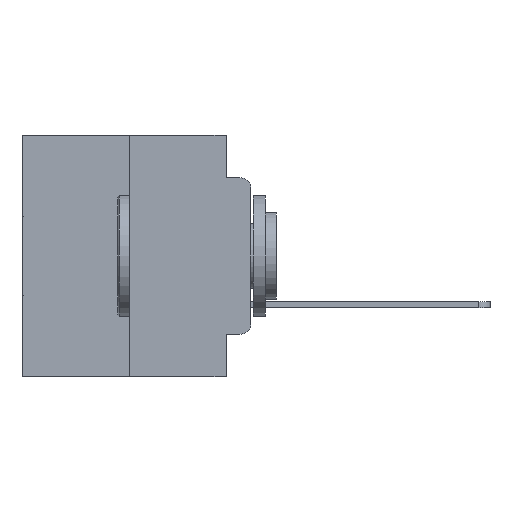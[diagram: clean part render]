
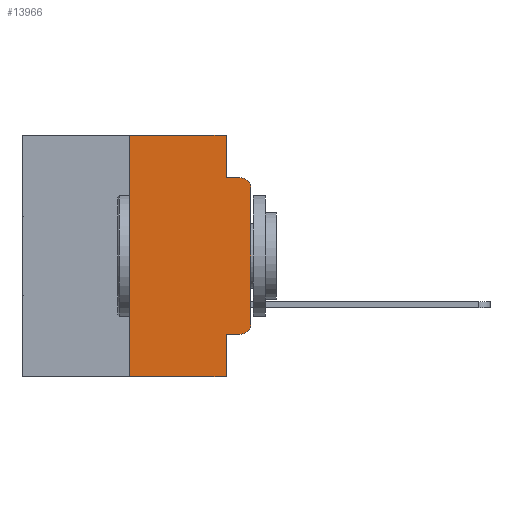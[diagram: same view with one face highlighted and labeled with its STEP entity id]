
A CAD part, left-side view. The second image highlights one B-rep face of the part: STEP entity #13966.
In plain terms, the highlighted planar face has unit normal (-1, 0, 0).
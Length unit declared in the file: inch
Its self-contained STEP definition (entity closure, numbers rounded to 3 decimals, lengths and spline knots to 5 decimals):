
#57 = VECTOR ( 'NONE', #1655, 39.37008 ) ;
#289 = CARTESIAN_POINT ( 'NONE',  ( 0., 0.051, 0. ) ) ;
#354 = DIRECTION ( 'NONE',  ( 1., 0., 0. ) ) ;
#413 = VERTEX_POINT ( 'NONE', #11187 ) ;
#441 = ORIENTED_EDGE ( 'NONE', *, *, #23303, .F. ) ;
#839 = EDGE_CURVE ( 'NONE', #23114, #413, #25658, .T. ) ;
#843 = VERTEX_POINT ( 'NONE', #8061 ) ;
#1576 = CARTESIAN_POINT ( 'NONE',  ( 0., 0., -0.3915 ) ) ;
#1613 = CARTESIAN_POINT ( 'NONE',  ( 0., 0.051, -0.0885 ) ) ;
#1655 = DIRECTION ( 'NONE',  ( 0., -1., 0. ) ) ;
#1890 = AXIS2_PLACEMENT_3D ( 'NONE', #11304, #27607, #13735 ) ;
#2071 = DIRECTION ( 'NONE',  ( 0., -1., 0. ) ) ;
#2687 = EDGE_CURVE ( 'NONE', #12668, #27361, #9742, .T. ) ;
#3389 = VERTEX_POINT ( 'NONE', #1576 ) ;
#4240 = VECTOR ( 'NONE', #24761, 39.37008 ) ;
#4814 = CARTESIAN_POINT ( 'NONE',  ( 0., 0.02, -0.1085 ) ) ;
#5627 = DIRECTION ( 'NONE',  ( 0., -1., 0. ) ) ;
#5711 = CARTESIAN_POINT ( 'NONE',  ( 0., 0.473, 0. ) ) ;
#6082 = AXIS2_PLACEMENT_3D ( 'NONE', #5711, #354, #18312 ) ;
#6217 = LINE ( 'NONE', #9698, #25439 ) ;
#6299 = EDGE_CURVE ( 'NONE', #11021, #9254, #6217, .T. ) ;
#7132 = CIRCLE ( 'NONE', #1890, 0.02 ) ;
#7500 = DIRECTION ( 'NONE',  ( 0., 0., -1. ) ) ;
#8061 = CARTESIAN_POINT ( 'NONE',  ( 0., 0.02, -0.4115 ) ) ;
#8072 = EDGE_CURVE ( 'NONE', #9254, #27324, #25543, .T. ) ;
#8433 = ORIENTED_EDGE ( 'NONE', *, *, #2687, .F. ) ;
#8852 = CARTESIAN_POINT ( 'NONE',  ( 0., 0.25, -0.5 ) ) ;
#8904 = CARTESIAN_POINT ( 'NONE',  ( 0., 0.051, 0. ) ) ;
#8998 = DIRECTION ( 'NONE',  ( 0., 0., -1. ) ) ;
#9254 = VERTEX_POINT ( 'NONE', #1613 ) ;
#9698 = CARTESIAN_POINT ( 'NONE',  ( 0., 0.051, 0. ) ) ;
#9742 = LINE ( 'NONE', #16015, #22557 ) ;
#9800 = EDGE_CURVE ( 'NONE', #26854, #27324, #20855, .T. ) ;
#10891 = ORIENTED_EDGE ( 'NONE', *, *, #839, .F. ) ;
#10941 = AXIS2_PLACEMENT_3D ( 'NONE', #4814, #22097, #7500 ) ;
#11021 = VERTEX_POINT ( 'NONE', #289 ) ;
#11187 = CARTESIAN_POINT ( 'NONE',  ( 0., 0.051, -0.5 ) ) ;
#11304 = CARTESIAN_POINT ( 'NONE',  ( 0., 0.02, -0.3915 ) ) ;
#11458 = EDGE_CURVE ( 'NONE', #3389, #26854, #26000, .T. ) ;
#11859 = EDGE_LOOP ( 'NONE', ( #30200, #12271, #13821, #30918, #441, #8433, #12361, #10891, #25355, #12493 ) ) ;
#12271 = ORIENTED_EDGE ( 'NONE', *, *, #9800, .T. ) ;
#12361 = ORIENTED_EDGE ( 'NONE', *, *, #19024, .T. ) ;
#12493 = ORIENTED_EDGE ( 'NONE', *, *, #29090, .T. ) ;
#12668 = VERTEX_POINT ( 'NONE', #8852 ) ;
#13551 = VECTOR ( 'NONE', #27024, 39.37008 ) ;
#13735 = DIRECTION ( 'NONE',  ( 0., 0., -1. ) ) ;
#13821 = ORIENTED_EDGE ( 'NONE', *, *, #8072, .F. ) ;
#13966 = ADVANCED_FACE ( 'NONE', ( #26443 ), #22870, .F. ) ;
#14552 = CARTESIAN_POINT ( 'NONE',  ( 0., 0.473, 0. ) ) ;
#16015 = CARTESIAN_POINT ( 'NONE',  ( 0., 0.25, 0. ) ) ;
#17396 = CARTESIAN_POINT ( 'NONE',  ( 0., 0.051, -0.0885 ) ) ;
#18013 = VECTOR ( 'NONE', #5627, 39.37008 ) ;
#18312 = DIRECTION ( 'NONE',  ( 0., 0., -1. ) ) ;
#18777 = LINE ( 'NONE', #20453, #18013 ) ;
#19024 = EDGE_CURVE ( 'NONE', #12668, #413, #23815, .T. ) ;
#20319 = LINE ( 'NONE', #14552, #57 ) ;
#20453 = CARTESIAN_POINT ( 'NONE',  ( 0., 0.051, -0.4115 ) ) ;
#20855 = CIRCLE ( 'NONE', #10941, 0.02 ) ;
#21591 = DIRECTION ( 'NONE',  ( 0., 0., 1. ) ) ;
#22097 = DIRECTION ( 'NONE',  ( -1., 0., 0. ) ) ;
#22548 = CARTESIAN_POINT ( 'NONE',  ( 0., 0.473, -0.5 ) ) ;
#22557 = VECTOR ( 'NONE', #21591, 39.37008 ) ;
#22870 = PLANE ( 'NONE',  #6082 ) ;
#23114 = VERTEX_POINT ( 'NONE', #25756 ) ;
#23303 = EDGE_CURVE ( 'NONE', #27361, #11021, #20319, .T. ) ;
#23815 = LINE ( 'NONE', #22548, #4240 ) ;
#24040 = CARTESIAN_POINT ( 'NONE',  ( 0., 0.25, 0. ) ) ;
#24761 = DIRECTION ( 'NONE',  ( 0., -1., 0. ) ) ;
#24958 = VECTOR ( 'NONE', #8998, 39.37008 ) ;
#24996 = CARTESIAN_POINT ( 'NONE',  ( 0., 0., 0. ) ) ;
#25355 = ORIENTED_EDGE ( 'NONE', *, *, #30494, .T. ) ;
#25439 = VECTOR ( 'NONE', #28298, 39.37008 ) ;
#25543 = LINE ( 'NONE', #17396, #30564 ) ;
#25658 = LINE ( 'NONE', #8904, #24958 ) ;
#25756 = CARTESIAN_POINT ( 'NONE',  ( 0., 0.051, -0.4115 ) ) ;
#26000 = LINE ( 'NONE', #24996, #13551 ) ;
#26443 = FACE_OUTER_BOUND ( 'NONE', #11859, .T. ) ;
#26854 = VERTEX_POINT ( 'NONE', #29371 ) ;
#27024 = DIRECTION ( 'NONE',  ( 0., 0., 1. ) ) ;
#27324 = VERTEX_POINT ( 'NONE', #30447 ) ;
#27361 = VERTEX_POINT ( 'NONE', #24040 ) ;
#27607 = DIRECTION ( 'NONE',  ( -1., 0., 0. ) ) ;
#28298 = DIRECTION ( 'NONE',  ( 0., 0., -1. ) ) ;
#29090 = EDGE_CURVE ( 'NONE', #843, #3389, #7132, .T. ) ;
#29371 = CARTESIAN_POINT ( 'NONE',  ( 0., 0., -0.1085 ) ) ;
#30200 = ORIENTED_EDGE ( 'NONE', *, *, #11458, .T. ) ;
#30447 = CARTESIAN_POINT ( 'NONE',  ( 0., 0.02, -0.0885 ) ) ;
#30494 = EDGE_CURVE ( 'NONE', #23114, #843, #18777, .T. ) ;
#30564 = VECTOR ( 'NONE', #2071, 39.37008 ) ;
#30918 = ORIENTED_EDGE ( 'NONE', *, *, #6299, .F. ) ;
